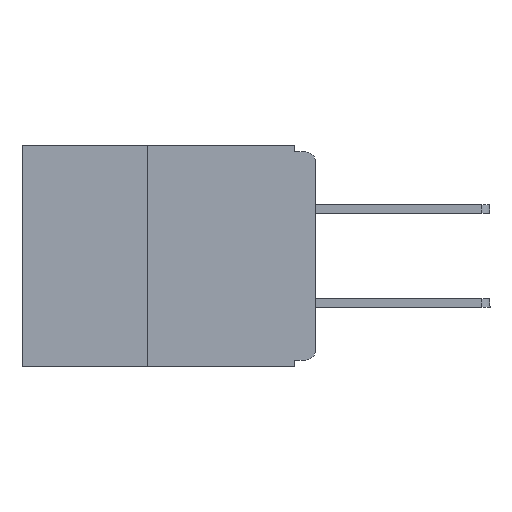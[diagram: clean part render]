
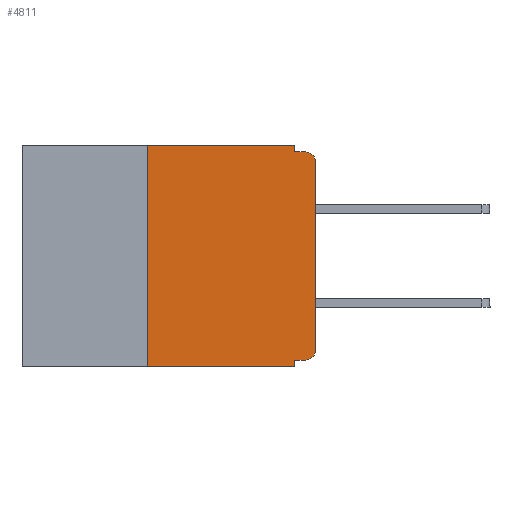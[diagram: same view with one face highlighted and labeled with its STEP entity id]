
A CAD part, left-side view. The second image highlights one B-rep face of the part: STEP entity #4811.
In plain terms, the highlighted planar face has unit normal (-1, 0, 0).
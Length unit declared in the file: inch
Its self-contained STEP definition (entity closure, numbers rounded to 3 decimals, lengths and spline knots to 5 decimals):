
#68 = EDGE_CURVE ( 'NONE', #11618, #10265, #3412, .T. ) ;
#71 = VERTEX_POINT ( 'NONE', #5624 ) ;
#192 = VECTOR ( 'NONE', #12352, 39.37008 ) ;
#230 = LINE ( 'NONE', #12362, #192 ) ;
#655 = EDGE_CURVE ( 'NONE', #3048, #1922, #2102, .T. ) ;
#883 = ORIENTED_EDGE ( 'NONE', *, *, #68, .F. ) ;
#1018 = DIRECTION ( 'NONE',  ( 0., 0., -1. ) ) ;
#1095 = DIRECTION ( 'NONE',  ( 0., 0., -1. ) ) ;
#1115 = VECTOR ( 'NONE', #7191, 39.37008 ) ;
#1209 = LINE ( 'NONE', #7452, #1115 ) ;
#1433 = DIRECTION ( 'NONE',  ( -1., 0., 0. ) ) ;
#1460 = CARTESIAN_POINT ( 'NONE',  ( 0., 0.015, -0.025 ) ) ;
#1600 = VECTOR ( 'NONE', #8630, 39.37008 ) ;
#1686 = VERTEX_POINT ( 'NONE', #11550 ) ;
#1800 = CIRCLE ( 'NONE', #5409, 0.015 ) ;
#1922 = VERTEX_POINT ( 'NONE', #6485 ) ;
#1927 = VERTEX_POINT ( 'NONE', #7027 ) ;
#1975 = PLANE ( 'NONE',  #6921 ) ;
#2003 = VECTOR ( 'NONE', #5452, 39.37008 ) ;
#2102 = LINE ( 'NONE', #3947, #2003 ) ;
#2394 = EDGE_CURVE ( 'NONE', #5555, #10265, #1800, .T. ) ;
#2454 = CARTESIAN_POINT ( 'NONE',  ( 0., 0.437, 0. ) ) ;
#2668 = CARTESIAN_POINT ( 'NONE',  ( 0., 0.031, -0.33 ) ) ;
#3048 = VERTEX_POINT ( 'NONE', #9458 ) ;
#3141 = CARTESIAN_POINT ( 'NONE',  ( 0., 0., -0.025 ) ) ;
#3397 = VECTOR ( 'NONE', #12188, 39.37008 ) ;
#3412 = LINE ( 'NONE', #3597, #3397 ) ;
#3597 = CARTESIAN_POINT ( 'NONE',  ( 0., 0., -0.01 ) ) ;
#3947 = CARTESIAN_POINT ( 'NONE',  ( 0., 0.437, 0. ) ) ;
#3972 = EDGE_CURVE ( 'NONE', #71, #3048, #7831, .T. ) ;
#3991 = VERTEX_POINT ( 'NONE', #9772 ) ;
#4041 = LINE ( 'NONE', #8453, #1600 ) ;
#4288 = EDGE_CURVE ( 'NONE', #9112, #1927, #7099, .T. ) ;
#4569 = ORIENTED_EDGE ( 'NONE', *, *, #7868, .F. ) ;
#4750 = CARTESIAN_POINT ( 'NONE',  ( 0., 0.031, -0.32 ) ) ;
#4811 = ADVANCED_FACE ( 'NONE', ( #6523 ), #1975, .F. ) ;
#4924 = CARTESIAN_POINT ( 'NONE',  ( 0., 0.015, -0.305 ) ) ;
#4993 = EDGE_CURVE ( 'NONE', #1686, #9112, #6137, .T. ) ;
#5052 = EDGE_CURVE ( 'NONE', #1686, #3991, #6001, .T. ) ;
#5078 = DIRECTION ( 'NONE',  ( 0., 0., -1. ) ) ;
#5121 = DIRECTION ( 'NONE',  ( -1., 0., 0. ) ) ;
#5409 = AXIS2_PLACEMENT_3D ( 'NONE', #1460, #1433, #1018 ) ;
#5452 = DIRECTION ( 'NONE',  ( 0., -1., 0. ) ) ;
#5555 = VERTEX_POINT ( 'NONE', #3141 ) ;
#5562 = DIRECTION ( 'NONE',  ( 0., 0., 1. ) ) ;
#5624 = CARTESIAN_POINT ( 'NONE',  ( 0., 0.25, -0.33 ) ) ;
#5670 = ORIENTED_EDGE ( 'NONE', *, *, #8938, .T. ) ;
#5869 = ORIENTED_EDGE ( 'NONE', *, *, #4993, .F. ) ;
#6001 = CIRCLE ( 'NONE', #6818, 0.015 ) ;
#6067 = VECTOR ( 'NONE', #10009, 39.37008 ) ;
#6117 = CARTESIAN_POINT ( 'NONE',  ( 0., 0.25, -0.33 ) ) ;
#6137 = LINE ( 'NONE', #8477, #6067 ) ;
#6485 = CARTESIAN_POINT ( 'NONE',  ( 0., 0.031, 0. ) ) ;
#6523 = FACE_OUTER_BOUND ( 'NONE', #7271, .T. ) ;
#6818 = AXIS2_PLACEMENT_3D ( 'NONE', #4924, #5121, #5078 ) ;
#6921 = AXIS2_PLACEMENT_3D ( 'NONE', #2454, #12417, #1095 ) ;
#7027 = CARTESIAN_POINT ( 'NONE',  ( 0., 0.031, -0.33 ) ) ;
#7099 = LINE ( 'NONE', #2668, #7163 ) ;
#7163 = VECTOR ( 'NONE', #11401, 39.37008 ) ;
#7191 = DIRECTION ( 'NONE',  ( 0., 0., 1. ) ) ;
#7271 = EDGE_LOOP ( 'NONE', ( #5670, #8775, #883, #4569, #7301, #7656, #7411, #7359, #5869, #8970 ) ) ;
#7301 = ORIENTED_EDGE ( 'NONE', *, *, #655, .F. ) ;
#7359 = ORIENTED_EDGE ( 'NONE', *, *, #4288, .F. ) ;
#7411 = ORIENTED_EDGE ( 'NONE', *, *, #9799, .T. ) ;
#7452 = CARTESIAN_POINT ( 'NONE',  ( 0., 0., 0. ) ) ;
#7656 = ORIENTED_EDGE ( 'NONE', *, *, #3972, .F. ) ;
#7831 = LINE ( 'NONE', #6117, #7844 ) ;
#7844 = VECTOR ( 'NONE', #5562, 39.37008 ) ;
#7868 = EDGE_CURVE ( 'NONE', #1922, #11618, #230, .T. ) ;
#7900 = CARTESIAN_POINT ( 'NONE',  ( 0., 0.015, -0.01 ) ) ;
#8453 = CARTESIAN_POINT ( 'NONE',  ( 0., 0.437, -0.33 ) ) ;
#8477 = CARTESIAN_POINT ( 'NONE',  ( 0., 0., -0.32 ) ) ;
#8630 = DIRECTION ( 'NONE',  ( 0., -1., 0. ) ) ;
#8775 = ORIENTED_EDGE ( 'NONE', *, *, #2394, .T. ) ;
#8938 = EDGE_CURVE ( 'NONE', #3991, #5555, #1209, .T. ) ;
#8970 = ORIENTED_EDGE ( 'NONE', *, *, #5052, .T. ) ;
#9112 = VERTEX_POINT ( 'NONE', #4750 ) ;
#9458 = CARTESIAN_POINT ( 'NONE',  ( 0., 0.25, 0. ) ) ;
#9772 = CARTESIAN_POINT ( 'NONE',  ( 0., 0., -0.305 ) ) ;
#9799 = EDGE_CURVE ( 'NONE', #71, #1927, #4041, .T. ) ;
#10009 = DIRECTION ( 'NONE',  ( 0., 1., 0. ) ) ;
#10265 = VERTEX_POINT ( 'NONE', #7900 ) ;
#11401 = DIRECTION ( 'NONE',  ( 0., 0., -1. ) ) ;
#11550 = CARTESIAN_POINT ( 'NONE',  ( 0., 0.015, -0.32 ) ) ;
#11618 = VERTEX_POINT ( 'NONE', #11743 ) ;
#11743 = CARTESIAN_POINT ( 'NONE',  ( 0., 0.031, -0.01 ) ) ;
#12188 = DIRECTION ( 'NONE',  ( 0., -1., 0. ) ) ;
#12352 = DIRECTION ( 'NONE',  ( 0., 0., -1. ) ) ;
#12362 = CARTESIAN_POINT ( 'NONE',  ( 0., 0.031, 0. ) ) ;
#12417 = DIRECTION ( 'NONE',  ( 1., 0., 0. ) ) ;
